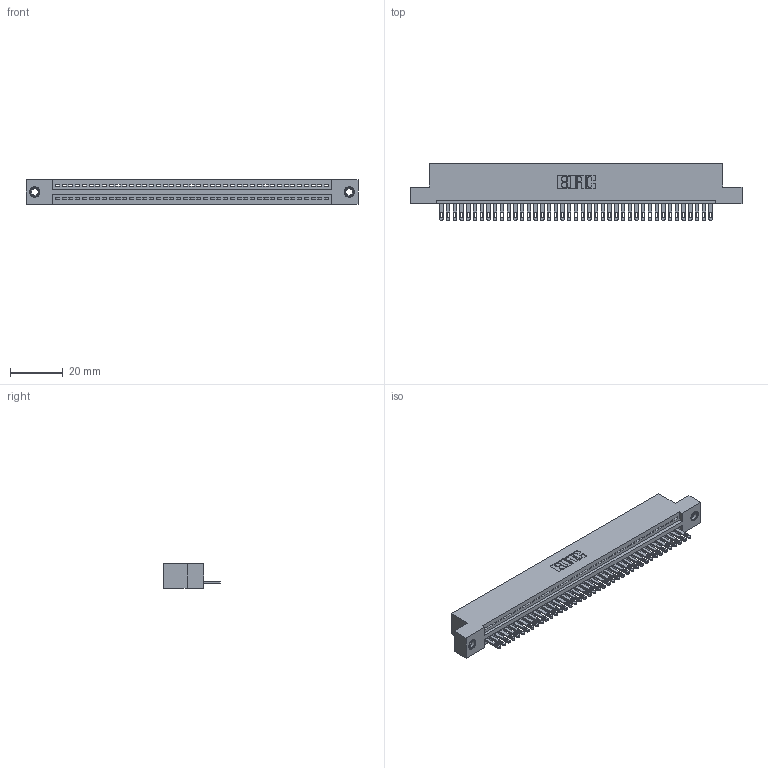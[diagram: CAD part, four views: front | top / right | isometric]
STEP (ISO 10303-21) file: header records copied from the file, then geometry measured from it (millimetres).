
FILE_DESCRIPTION (( 'STEP AP203' ), '1' );
FILE_NAME ('345-041-500-107.STEP', '2018-09-05T06:39:36', ( '' ), ( '' ), 'SwSTEP 2.0', 'SolidWorks 2016', '' );
FILE_SCHEMA (( 'CONFIG_CONTROL_DESIGN' ));
Length unit declared in the file: inch
Products named in the file (4): 345 Part_Flush Mounting Lugs - 0.156 Dia-TI; 345-292-001_345-293-100; 345-250-001_345-250-005-103; 345-041-500-107
Assembly tree (44 placements, depth 2):
  345-041-500-107
    345 Part_Flush Mounting Lugs - 0.156 Dia-TI
    345-292-001_345-293-100  x41
    345-250-001_345-250-005-103  x2
Bounding box: 125.35 x 21.51 x 9.4 mm (x, y, z)
Volume: 587.3 mm3; surface area: 15917.9 mm2
Topology: 43 solids, 44 shells, 2399 faces, 7365 edges, 4902 vertices
Faces by surface type: plane 1505, cylinder 878, cone 12, torus 4
Entity records: 32108 total; most frequent: CARTESIAN_POINT 5542, ORIENTED_EDGE 5510, DIRECTION 4871, EDGE_CURVE 2755, VECTOR 2435, LINE 2435, VERTEX_POINT 1832, AXIS2_PLACEMENT_3D 1218
